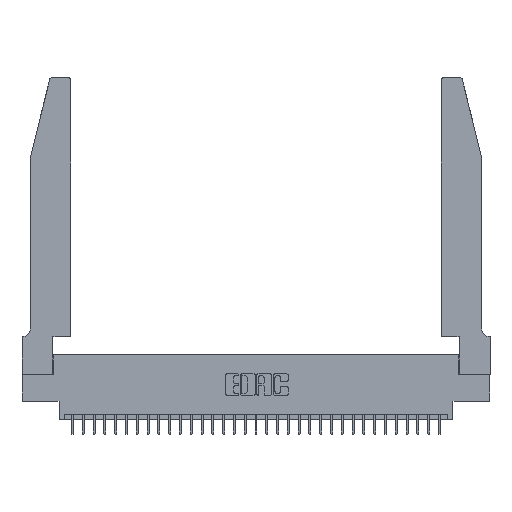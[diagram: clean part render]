
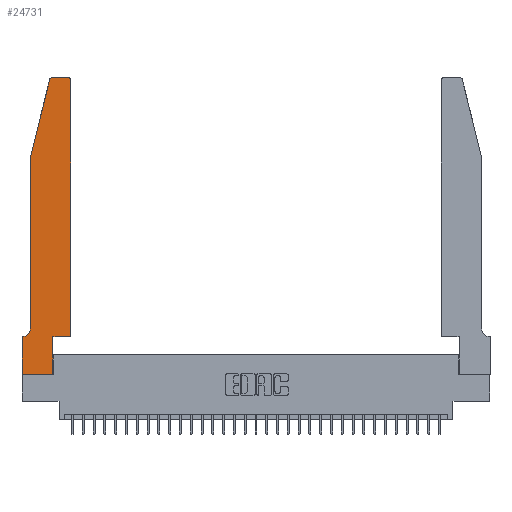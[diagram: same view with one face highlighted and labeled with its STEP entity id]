
A CAD part, top view. The second image highlights one B-rep face of the part: STEP entity #24731.
In plain terms, the highlighted planar face has unit normal (0, 0, 1).
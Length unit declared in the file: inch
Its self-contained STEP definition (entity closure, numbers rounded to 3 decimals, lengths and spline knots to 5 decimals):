
#381 = VERTEX_POINT ( 'NONE', #33119 ) ;
#485 = ORIENTED_EDGE ( 'NONE', *, *, #5919, .T. ) ;
#734 = CARTESIAN_POINT ( 'NONE',  ( 0.284, 2.72, 0.37 ) ) ;
#1512 = PLANE ( 'NONE',  #22564 ) ;
#2094 = EDGE_CURVE ( 'NONE', #17604, #22167, #14309, .T. ) ;
#2257 = CARTESIAN_POINT ( 'NONE',  ( 0.0755, 0.42, 0.37 ) ) ;
#3354 = DIRECTION ( 'NONE',  ( -1., 0., 0. ) ) ;
#3540 = FACE_OUTER_BOUND ( 'NONE', #6520, .T. ) ;
#4050 = VECTOR ( 'NONE', #3354, 39.37008 ) ;
#5376 = VERTEX_POINT ( 'NONE', #17399 ) ;
#5919 = EDGE_CURVE ( 'NONE', #18652, #24297, #18019, .T. ) ;
#6299 = AXIS2_PLACEMENT_3D ( 'NONE', #23302, #13290, #28391 ) ;
#6520 = EDGE_LOOP ( 'NONE', ( #7149, #9737, #32513, #485, #24421, #29335, #22558, #31034, #10560, #23900, #29386, #26252 ) ) ;
#6564 = DIRECTION ( 'NONE',  ( 1., 0., 0. ) ) ;
#7149 = ORIENTED_EDGE ( 'NONE', *, *, #21689, .T. ) ;
#7616 = VECTOR ( 'NONE', #10041, 39.37008 ) ;
#8742 = EDGE_CURVE ( 'NONE', #15034, #5376, #14135, .T. ) ;
#8825 = DIRECTION ( 'NONE',  ( 1., 0., 0. ) ) ;
#9393 = EDGE_CURVE ( 'NONE', #32468, #29907, #20421, .T. ) ;
#9497 = CARTESIAN_POINT ( 'NONE',  ( 0.4205, 2.72, 0.37 ) ) ;
#9737 = ORIENTED_EDGE ( 'NONE', *, *, #8742, .T. ) ;
#9922 = DIRECTION ( 'NONE',  ( 0., 1., 0. ) ) ;
#10041 = DIRECTION ( 'NONE',  ( 0., 1., 0. ) ) ;
#10367 = LINE ( 'NONE', #17492, #25738 ) ;
#10560 = ORIENTED_EDGE ( 'NONE', *, *, #21920, .T. ) ;
#10562 = CARTESIAN_POINT ( 'NONE',  ( 0.4505, 2.72, 0.37 ) ) ;
#10566 = DIRECTION ( 'NONE',  ( -1., 0., 0. ) ) ;
#12425 = CARTESIAN_POINT ( 'NONE',  ( 0.2865, 0.35, 0.37 ) ) ;
#13116 = LINE ( 'NONE', #23455, #29667 ) ;
#13290 = DIRECTION ( 'NONE',  ( 0., 0., -1. ) ) ;
#13582 = CARTESIAN_POINT ( 'NONE',  ( 0.0755, 2., 0.37 ) ) ;
#14007 = VERTEX_POINT ( 'NONE', #20551 ) ;
#14135 = CIRCLE ( 'NONE', #31963, 0.03 ) ;
#14309 = LINE ( 'NONE', #21942, #32975 ) ;
#14481 = DIRECTION ( 'NONE',  ( 0., -1., 0. ) ) ;
#15034 = VERTEX_POINT ( 'NONE', #21637 ) ;
#15116 = DIRECTION ( 'NONE',  ( 1., 0., 0. ) ) ;
#15656 = CARTESIAN_POINT ( 'NONE',  ( 0.4505, 0.35, 0.37 ) ) ;
#15840 = LINE ( 'NONE', #26376, #4050 ) ;
#17399 = CARTESIAN_POINT ( 'NONE',  ( 0.25487, 2.72718, 0.37 ) ) ;
#17492 = CARTESIAN_POINT ( 'NONE',  ( 0.4505, 0.35, 0.37 ) ) ;
#17604 = VERTEX_POINT ( 'NONE', #28747 ) ;
#17635 = CIRCLE ( 'NONE', #6299, 0.07 ) ;
#18019 = LINE ( 'NONE', #25848, #26260 ) ;
#18089 = DIRECTION ( 'NONE',  ( -0.239, -0.971, 0. ) ) ;
#18158 = CARTESIAN_POINT ( 'NONE',  ( 0., 0., 0.37 ) ) ;
#18487 = VECTOR ( 'NONE', #9922, 39.37008 ) ;
#18651 = DIRECTION ( 'NONE',  ( 0., 0., 1. ) ) ;
#18652 = VERTEX_POINT ( 'NONE', #13582 ) ;
#19904 = CARTESIAN_POINT ( 'NONE',  ( 0.4505, 0.35, 0.37 ) ) ;
#20421 = LINE ( 'NONE', #19904, #18487 ) ;
#20551 = CARTESIAN_POINT ( 'NONE',  ( 0.4205, 2.75, 0.37 ) ) ;
#21637 = CARTESIAN_POINT ( 'NONE',  ( 0.284, 2.75, 0.37 ) ) ;
#21689 = EDGE_CURVE ( 'NONE', #14007, #15034, #13116, .T. ) ;
#21846 = AXIS2_PLACEMENT_3D ( 'NONE', #9497, #33335, #30654 ) ;
#21861 = VERTEX_POINT ( 'NONE', #12425 ) ;
#21920 = EDGE_CURVE ( 'NONE', #381, #21861, #22584, .T. ) ;
#21942 = CARTESIAN_POINT ( 'NONE',  ( 0., 0., 0.37 ) ) ;
#21958 = CARTESIAN_POINT ( 'NONE',  ( 0., 0.35, 0.37 ) ) ;
#22167 = VERTEX_POINT ( 'NONE', #26966 ) ;
#22558 = ORIENTED_EDGE ( 'NONE', *, *, #2094, .T. ) ;
#22564 = AXIS2_PLACEMENT_3D ( 'NONE', #21958, #24186, #6564 ) ;
#22584 = LINE ( 'NONE', #22905, #7616 ) ;
#22834 = VECTOR ( 'NONE', #18089, 39.37008 ) ;
#22905 = CARTESIAN_POINT ( 'NONE',  ( 0.2865, 0.35, 0.37 ) ) ;
#23283 = DIRECTION ( 'NONE',  ( 0., -1., 0. ) ) ;
#23302 = CARTESIAN_POINT ( 'NONE',  ( 0.0055, 0.42, 0.37 ) ) ;
#23455 = CARTESIAN_POINT ( 'NONE',  ( 0.2605, 2.75, 0.37 ) ) ;
#23900 = ORIENTED_EDGE ( 'NONE', *, *, #31381, .T. ) ;
#23935 = EDGE_CURVE ( 'NONE', #22167, #381, #31017, .T. ) ;
#24186 = DIRECTION ( 'NONE',  ( 0., 0., 1. ) ) ;
#24297 = VERTEX_POINT ( 'NONE', #2257 ) ;
#24421 = ORIENTED_EDGE ( 'NONE', *, *, #32382, .T. ) ;
#24731 = ADVANCED_FACE ( 'NONE', ( #3540 ), #1512, .T. ) ;
#24785 = CARTESIAN_POINT ( 'NONE',  ( 0.0055, 0.35, 0.37 ) ) ;
#25423 = LINE ( 'NONE', #28275, #22834 ) ;
#25738 = VECTOR ( 'NONE', #15116, 39.37008 ) ;
#25848 = CARTESIAN_POINT ( 'NONE',  ( 0.0755, 2., 0.37 ) ) ;
#25905 = EDGE_CURVE ( 'NONE', #5376, #18652, #25423, .T. ) ;
#26252 = ORIENTED_EDGE ( 'NONE', *, *, #30426, .T. ) ;
#26260 = VECTOR ( 'NONE', #23283, 39.37008 ) ;
#26376 = CARTESIAN_POINT ( 'NONE',  ( 0.0755, 0.35, 0.37 ) ) ;
#26966 = CARTESIAN_POINT ( 'NONE',  ( 0., 0., 0.37 ) ) ;
#27225 = VERTEX_POINT ( 'NONE', #24785 ) ;
#28260 = EDGE_CURVE ( 'NONE', #27225, #17604, #15840, .T. ) ;
#28275 = CARTESIAN_POINT ( 'NONE',  ( 0.0755, 2., 0.37 ) ) ;
#28391 = DIRECTION ( 'NONE',  ( -1., 0., 0. ) ) ;
#28747 = CARTESIAN_POINT ( 'NONE',  ( 0., 0.35, 0.37 ) ) ;
#29241 = VECTOR ( 'NONE', #30534, 39.37008 ) ;
#29335 = ORIENTED_EDGE ( 'NONE', *, *, #28260, .T. ) ;
#29386 = ORIENTED_EDGE ( 'NONE', *, *, #9393, .T. ) ;
#29667 = VECTOR ( 'NONE', #10566, 39.37008 ) ;
#29907 = VERTEX_POINT ( 'NONE', #10562 ) ;
#30426 = EDGE_CURVE ( 'NONE', #29907, #14007, #32109, .T. ) ;
#30534 = DIRECTION ( 'NONE',  ( 1., 0., 0. ) ) ;
#30654 = DIRECTION ( 'NONE',  ( 1., 0., 0. ) ) ;
#31017 = LINE ( 'NONE', #18158, #29241 ) ;
#31034 = ORIENTED_EDGE ( 'NONE', *, *, #23935, .T. ) ;
#31381 = EDGE_CURVE ( 'NONE', #21861, #32468, #10367, .T. ) ;
#31963 = AXIS2_PLACEMENT_3D ( 'NONE', #734, #18651, #8825 ) ;
#32109 = CIRCLE ( 'NONE', #21846, 0.03 ) ;
#32382 = EDGE_CURVE ( 'NONE', #24297, #27225, #17635, .T. ) ;
#32468 = VERTEX_POINT ( 'NONE', #15656 ) ;
#32513 = ORIENTED_EDGE ( 'NONE', *, *, #25905, .T. ) ;
#32975 = VECTOR ( 'NONE', #14481, 39.37008 ) ;
#33119 = CARTESIAN_POINT ( 'NONE',  ( 0.2865, 0., 0.37 ) ) ;
#33335 = DIRECTION ( 'NONE',  ( 0., 0., 1. ) ) ;
